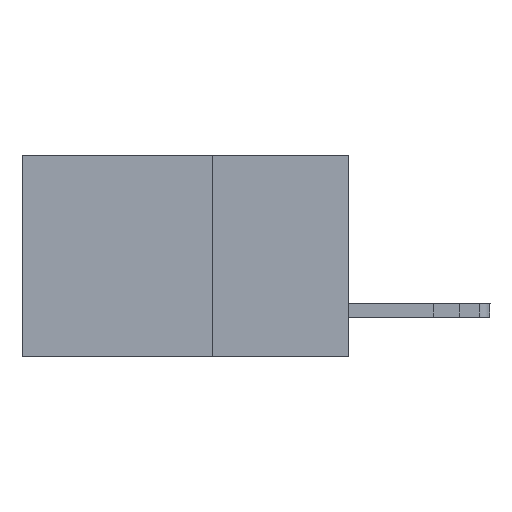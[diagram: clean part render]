
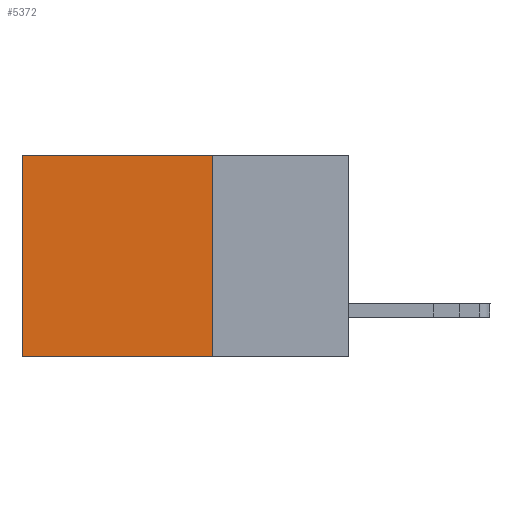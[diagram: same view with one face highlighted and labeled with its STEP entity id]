
A CAD part, left-side view. The second image highlights one B-rep face of the part: STEP entity #5372.
In plain terms, the highlighted planar face has unit normal (-1, 0, 0).
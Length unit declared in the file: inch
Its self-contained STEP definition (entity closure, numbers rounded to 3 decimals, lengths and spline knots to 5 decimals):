
#230 = CARTESIAN_POINT ( 'NONE',  ( 0.298, 0.6, 0. ) ) ;
#856 = EDGE_CURVE ( 'NONE', #6182, #8257, #9176, .T. ) ;
#991 = EDGE_LOOP ( 'NONE', ( #11729, #3484, #2831, #10251 ) ) ;
#1248 = VECTOR ( 'NONE', #2647, 39.37008 ) ;
#1838 = EDGE_CURVE ( 'NONE', #7804, #11484, #3748, .T. ) ;
#1897 = VECTOR ( 'NONE', #11547, 39.37008 ) ;
#2344 = LINE ( 'NONE', #10713, #10607 ) ;
#2647 = DIRECTION ( 'NONE',  ( 0., 0., -1. ) ) ;
#2831 = ORIENTED_EDGE ( 'NONE', *, *, #6632, .F. ) ;
#3484 = ORIENTED_EDGE ( 'NONE', *, *, #856, .F. ) ;
#3649 = DIRECTION ( 'NONE',  ( 1., 0., 0. ) ) ;
#3748 = LINE ( 'NONE', #9500, #1897 ) ;
#4289 = VECTOR ( 'NONE', #9153, 39.37008 ) ;
#4922 = CARTESIAN_POINT ( 'NONE',  ( 0.298, 0.25, 0. ) ) ;
#5372 = ADVANCED_FACE ( 'NONE', ( #8573 ), #12184, .F. ) ;
#5522 = CARTESIAN_POINT ( 'NONE',  ( 0.298, 0.25, -0.37 ) ) ;
#6182 = VERTEX_POINT ( 'NONE', #5522 ) ;
#6632 = EDGE_CURVE ( 'NONE', #7804, #6182, #9031, .T. ) ;
#7455 = AXIS2_PLACEMENT_3D ( 'NONE', #11221, #3649, #13210 ) ;
#7804 = VERTEX_POINT ( 'NONE', #9970 ) ;
#8257 = VERTEX_POINT ( 'NONE', #12082 ) ;
#8573 = FACE_OUTER_BOUND ( 'NONE', #991, .T. ) ;
#9031 = LINE ( 'NONE', #4922, #1248 ) ;
#9153 = DIRECTION ( 'NONE',  ( 0., 1., 0. ) ) ;
#9176 = LINE ( 'NONE', #10350, #4289 ) ;
#9500 = CARTESIAN_POINT ( 'NONE',  ( 0.298, 0.25, 0. ) ) ;
#9970 = CARTESIAN_POINT ( 'NONE',  ( 0.298, 0.25, 0. ) ) ;
#10251 = ORIENTED_EDGE ( 'NONE', *, *, #1838, .T. ) ;
#10350 = CARTESIAN_POINT ( 'NONE',  ( 0.298, 0.25, -0.37 ) ) ;
#10607 = VECTOR ( 'NONE', #13935, 39.37008 ) ;
#10713 = CARTESIAN_POINT ( 'NONE',  ( 0.298, 0.6, 0. ) ) ;
#11221 = CARTESIAN_POINT ( 'NONE',  ( 0.298, 0.25, 0. ) ) ;
#11484 = VERTEX_POINT ( 'NONE', #230 ) ;
#11547 = DIRECTION ( 'NONE',  ( 0., 1., 0. ) ) ;
#11729 = ORIENTED_EDGE ( 'NONE', *, *, #12373, .T. ) ;
#12082 = CARTESIAN_POINT ( 'NONE',  ( 0.298, 0.6, -0.37 ) ) ;
#12184 = PLANE ( 'NONE',  #7455 ) ;
#12373 = EDGE_CURVE ( 'NONE', #11484, #8257, #2344, .T. ) ;
#13210 = DIRECTION ( 'NONE',  ( 0., 0., -1. ) ) ;
#13935 = DIRECTION ( 'NONE',  ( 0., 0., -1. ) ) ;
